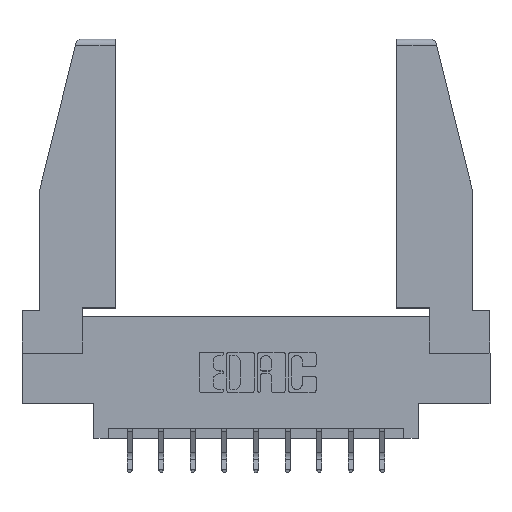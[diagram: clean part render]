
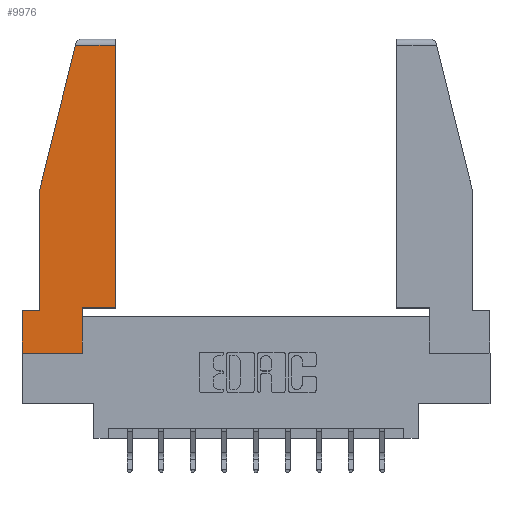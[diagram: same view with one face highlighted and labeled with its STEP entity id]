
A CAD part, top view. The second image highlights one B-rep face of the part: STEP entity #9976.
In plain terms, the highlighted planar face has unit normal (0, 0, 1).
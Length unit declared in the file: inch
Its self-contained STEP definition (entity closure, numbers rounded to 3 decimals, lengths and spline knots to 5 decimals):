
#150 = FACE_OUTER_BOUND ( 'NONE', #11660, .T. ) ;
#233 = ORIENTED_EDGE ( 'NONE', *, *, #4348, .T. ) ;
#412 = VECTOR ( 'NONE', #13520, 39.37008 ) ;
#442 = VERTEX_POINT ( 'NONE', #12376 ) ;
#505 = VECTOR ( 'NONE', #5390, 39.37008 ) ;
#959 = CARTESIAN_POINT ( 'NONE',  ( 0.2636, 1.52, 0. ) ) ;
#1018 = LINE ( 'NONE', #2140, #2026 ) ;
#1106 = DIRECTION ( 'NONE',  ( 0., 1., 0. ) ) ;
#1345 = ORIENTED_EDGE ( 'NONE', *, *, #5308, .T. ) ;
#1533 = EDGE_CURVE ( 'NONE', #11316, #9703, #5030, .T. ) ;
#1574 = VECTOR ( 'NONE', #1106, 39.37008 ) ;
#1872 = CARTESIAN_POINT ( 'NONE',  ( 0.297, 0.223, 0. ) ) ;
#2026 = VECTOR ( 'NONE', #4533, 39.37008 ) ;
#2080 = AXIS2_PLACEMENT_3D ( 'NONE', #12111, #6629, #2159 ) ;
#2115 = VECTOR ( 'NONE', #6255, 39.37008 ) ;
#2140 = CARTESIAN_POINT ( 'NONE',  ( 0.297, 0.223, 0. ) ) ;
#2159 = DIRECTION ( 'NONE',  ( 1., 0., 0. ) ) ;
#2222 = EDGE_CURVE ( 'NONE', #5775, #11316, #6039, .T. ) ;
#2364 = LINE ( 'NONE', #13984, #505 ) ;
#2431 = CARTESIAN_POINT ( 'NONE',  ( 0.461, 0.223, 0. ) ) ;
#3069 = ORIENTED_EDGE ( 'NONE', *, *, #11504, .T. ) ;
#3136 = DIRECTION ( 'NONE',  ( -1., 0., 0. ) ) ;
#3289 = LINE ( 'NONE', #9816, #1574 ) ;
#3997 = VERTEX_POINT ( 'NONE', #12611 ) ;
#4028 = CARTESIAN_POINT ( 'NONE',  ( 0.086, 0.21, 0. ) ) ;
#4108 = DIRECTION ( 'NONE',  ( 0., -1., 0. ) ) ;
#4161 = CARTESIAN_POINT ( 'NONE',  ( 0., 0.21, 0. ) ) ;
#4348 = EDGE_CURVE ( 'NONE', #9703, #13951, #2364, .T. ) ;
#4406 = PLANE ( 'NONE',  #2080 ) ;
#4533 = DIRECTION ( 'NONE',  ( 1., 0., 0. ) ) ;
#5030 = LINE ( 'NONE', #11561, #2115 ) ;
#5308 = EDGE_CURVE ( 'NONE', #7717, #5775, #9363, .T. ) ;
#5335 = VERTEX_POINT ( 'NONE', #12994 ) ;
#5390 = DIRECTION ( 'NONE',  ( 0., -1., 0. ) ) ;
#5639 = CARTESIAN_POINT ( 'NONE',  ( 0.461, 1.52, 0. ) ) ;
#5775 = VERTEX_POINT ( 'NONE', #5639 ) ;
#5811 = CARTESIAN_POINT ( 'NONE',  ( 0.086, 0.8, 0. ) ) ;
#5992 = LINE ( 'NONE', #9038, #8559 ) ;
#6039 = LINE ( 'NONE', #10301, #412 ) ;
#6255 = DIRECTION ( 'NONE',  ( -0.239, -0.971, 0. ) ) ;
#6422 = CARTESIAN_POINT ( 'NONE',  ( 0., 0.21, 0. ) ) ;
#6436 = VECTOR ( 'NONE', #3136, 39.37008 ) ;
#6629 = DIRECTION ( 'NONE',  ( 0., 0., 1. ) ) ;
#6657 = VERTEX_POINT ( 'NONE', #1872 ) ;
#7043 = ORIENTED_EDGE ( 'NONE', *, *, #9539, .T. ) ;
#7098 = EDGE_CURVE ( 'NONE', #13951, #442, #9137, .T. ) ;
#7146 = ORIENTED_EDGE ( 'NONE', *, *, #1533, .T. ) ;
#7352 = ORIENTED_EDGE ( 'NONE', *, *, #9485, .T. ) ;
#7500 = DIRECTION ( 'NONE',  ( 0., 1., 0. ) ) ;
#7717 = VERTEX_POINT ( 'NONE', #2431 ) ;
#7974 = ORIENTED_EDGE ( 'NONE', *, *, #2222, .T. ) ;
#8559 = VECTOR ( 'NONE', #10112, 39.37008 ) ;
#9026 = VECTOR ( 'NONE', #7500, 39.37008 ) ;
#9038 = CARTESIAN_POINT ( 'NONE',  ( 0., 0., 0. ) ) ;
#9137 = LINE ( 'NONE', #6422, #6436 ) ;
#9363 = LINE ( 'NONE', #12887, #9026 ) ;
#9485 = EDGE_CURVE ( 'NONE', #442, #5335, #12083, .T. ) ;
#9539 = EDGE_CURVE ( 'NONE', #6657, #7717, #1018, .T. ) ;
#9703 = VERTEX_POINT ( 'NONE', #5811 ) ;
#9816 = CARTESIAN_POINT ( 'NONE',  ( 0.297, 0., 0. ) ) ;
#9976 = ADVANCED_FACE ( 'NONE', ( #150 ), #4406, .T. ) ;
#10112 = DIRECTION ( 'NONE',  ( 1., 0., 0. ) ) ;
#10301 = CARTESIAN_POINT ( 'NONE',  ( 0., 1.52, 0. ) ) ;
#11316 = VERTEX_POINT ( 'NONE', #959 ) ;
#11398 = VECTOR ( 'NONE', #4108, 39.37008 ) ;
#11401 = ORIENTED_EDGE ( 'NONE', *, *, #7098, .T. ) ;
#11504 = EDGE_CURVE ( 'NONE', #3997, #6657, #3289, .T. ) ;
#11561 = CARTESIAN_POINT ( 'NONE',  ( 0.271, 1.55, 0. ) ) ;
#11660 = EDGE_LOOP ( 'NONE', ( #1345, #7974, #7146, #233, #11401, #7352, #13991, #3069, #7043 ) ) ;
#12083 = LINE ( 'NONE', #4161, #11398 ) ;
#12111 = CARTESIAN_POINT ( 'NONE',  ( 0., 0., 0. ) ) ;
#12376 = CARTESIAN_POINT ( 'NONE',  ( 0., 0.21, 0. ) ) ;
#12611 = CARTESIAN_POINT ( 'NONE',  ( 0.297, 0., 0. ) ) ;
#12887 = CARTESIAN_POINT ( 'NONE',  ( 0.461, 0.223, 0. ) ) ;
#12994 = CARTESIAN_POINT ( 'NONE',  ( 0., 0., 0. ) ) ;
#13520 = DIRECTION ( 'NONE',  ( -1., 0., 0. ) ) ;
#13774 = EDGE_CURVE ( 'NONE', #5335, #3997, #5992, .T. ) ;
#13951 = VERTEX_POINT ( 'NONE', #4028 ) ;
#13984 = CARTESIAN_POINT ( 'NONE',  ( 0.086, 0.8, 0. ) ) ;
#13991 = ORIENTED_EDGE ( 'NONE', *, *, #13774, .T. ) ;
